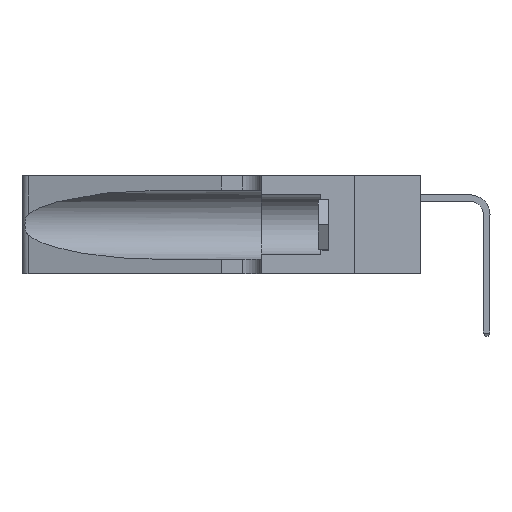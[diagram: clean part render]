
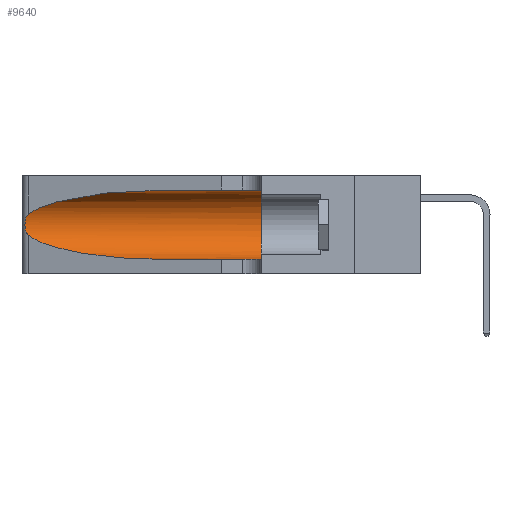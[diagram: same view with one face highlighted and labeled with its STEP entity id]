
A CAD part, left-side view. The second image highlights one B-rep face of the part: STEP entity #9640.
In plain terms, the highlighted cylindrical face has radius 3.308 mm (diameter 6.617 mm), a partial arc.
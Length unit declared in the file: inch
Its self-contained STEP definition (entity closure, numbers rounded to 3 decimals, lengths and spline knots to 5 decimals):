
#336 = CARTESIAN_POINT ( 'NONE',  ( 0.25487, 1.22718, 0.22369 ) ) ;
#427 = DIRECTION ( 'NONE',  ( 0., 0., 1. ) ) ;
#864 = CARTESIAN_POINT ( 'NONE',  ( 0.25487, 1.22718, 0.22369 ) ) ;
#1124 = AXIS2_PLACEMENT_3D ( 'NONE', #34029, #17379, #427 ) ;
#2568 = CARTESIAN_POINT ( 'NONE',  ( 0.25789, 1.23486, 0.15765 ) ) ;
#3024 = EDGE_CURVE ( 'NONE', #29465, #32838, #11775, .T. ) ;
#3069 = CARTESIAN_POINT ( 'NONE',  ( 0.1305, 0.72297, 0.31525 ) ) ;
#4039 = CARTESIAN_POINT ( 'NONE',  ( 0.1305, 0.72297, 0.05475 ) ) ;
#4772 = CARTESIAN_POINT ( 'NONE',  ( 0.1305, 0.72297, 0.05475 ) ) ;
#4785 = VECTOR ( 'NONE', #34734, 39.37008 ) ;
#5292 = CARTESIAN_POINT ( 'NONE',  ( 0.25555, 1.22994, 0.2215 ) ) ;
#5407 = CARTESIAN_POINT ( 'NONE',  ( 0.25555, 1.22993, 0.14849 ) ) ;
#6448 = ORIENTED_EDGE ( 'NONE', *, *, #29669, .T. ) ;
#6559 = CIRCLE ( 'NONE', #1124, 0.13025 ) ;
#8004 = CARTESIAN_POINT ( 'NONE',  ( 0.25487, 1.22718, 0.22369 ) ) ;
#8681 = ORIENTED_EDGE ( 'NONE', *, *, #9559, .F. ) ;
#8754 = CARTESIAN_POINT ( 'NONE',  ( 0.18966, 0.96281, 0.31525 ) ) ;
#9010 = VERTEX_POINT ( 'NONE', #864 ) ;
#9559 = EDGE_CURVE ( 'NONE', #32838, #14197, #6559, .T. ) ;
#9619 = CARTESIAN_POINT ( 'NONE',  ( 0.2373, 1.15595, 0.08982 ) ) ;
#9640 = ADVANCED_FACE ( 'NONE', ( #32488 ), #10149, .F. ) ;
#10149 = CYLINDRICAL_SURFACE ( 'NONE', #16273, 0.13025 ) ;
#10292 = EDGE_CURVE ( 'NONE', #32568, #14197, #32848, .T. ) ;
#10497 = DIRECTION ( 'NONE',  ( 0., -1., 0. ) ) ;
#10960 = CARTESIAN_POINT ( 'NONE',  ( 0.25787, 1.23484, 0.2124 ) ) ;
#11775 = LINE ( 'NONE', #19025, #25821 ) ;
#12058 = CARTESIAN_POINT ( 'NONE',  ( 0.1305, 1.61858, 0.185 ) ) ;
#13831 = CARTESIAN_POINT ( 'NONE',  ( 0.26018, 1.23835, 0.19895 ) ) ;
#14197 = VERTEX_POINT ( 'NONE', #29158 ) ;
#16273 = AXIS2_PLACEMENT_3D ( 'NONE', #12058, #31618, #26050 ) ;
#16666 = CARTESIAN_POINT ( 'NONE',  ( 0.26075, 1.23896, 0.178 ) ) ;
#16757 =( BOUNDED_CURVE ( )  B_SPLINE_CURVE ( 3, ( #3069, #8754, #17287, #336 ),
 .UNSPECIFIED., .F., .T. ) 
 B_SPLINE_CURVE_WITH_KNOTS ( ( 4, 4 ),
 ( 1.5708, 2.84003 ),
 .UNSPECIFIED. ) 
 CURVE ( )  GEOMETRIC_REPRESENTATION_ITEM ( )  RATIONAL_B_SPLINE_CURVE ( ( 1., 0.87, 0.87, 1. ) ) 
 REPRESENTATION_ITEM ( '' )  );
#17287 = CARTESIAN_POINT ( 'NONE',  ( 0.2373, 1.15595, 0.28018 ) ) ;
#17379 = DIRECTION ( 'NONE',  ( 0., 1., 0. ) ) ;
#17400 = ORIENTED_EDGE ( 'NONE', *, *, #22391, .T. ) ;
#19025 = CARTESIAN_POINT ( 'NONE',  ( 0.1305, 1.61858, 0.31525 ) ) ;
#19323 = EDGE_CURVE ( 'NONE', #9010, #26788, #35095, .T. ) ;
#19490 = CARTESIAN_POINT ( 'NONE',  ( 0.25856, 1.23593, 0.16098 ) ) ;
#20527 =( BOUNDED_CURVE ( )  B_SPLINE_CURVE ( 3, ( #32010, #9619, #20956, #4039 ),
 .UNSPECIFIED., .F., .F. ) 
 B_SPLINE_CURVE_WITH_KNOTS ( ( 4, 4 ),
 ( 3.44316, 4.71239 ),
 .UNSPECIFIED. ) 
 CURVE ( )  GEOMETRIC_REPRESENTATION_ITEM ( )  RATIONAL_B_SPLINE_CURVE ( ( 1., 0.87, 0.87, 1. ) ) 
 REPRESENTATION_ITEM ( '' )  );
#20602 = ORIENTED_EDGE ( 'NONE', *, *, #3024, .F. ) ;
#20956 = CARTESIAN_POINT ( 'NONE',  ( 0.18966, 0.96281, 0.05475 ) ) ;
#22290 = CARTESIAN_POINT ( 'NONE',  ( 0.25639, 1.23186, 0.15144 ) ) ;
#22391 = EDGE_CURVE ( 'NONE', #29465, #9010, #16757, .T. ) ;
#22992 = EDGE_LOOP ( 'NONE', ( #17400, #27299, #6448, #25802, #8681, #20602 ) ) ;
#24677 = CARTESIAN_POINT ( 'NONE',  ( 0.25487, 1.22718, 0.14631 ) ) ;
#25096 = CARTESIAN_POINT ( 'NONE',  ( 0.25487, 1.22718, 0.14631 ) ) ;
#25802 = ORIENTED_EDGE ( 'NONE', *, *, #10292, .T. ) ;
#25821 = VECTOR ( 'NONE', #10497, 39.37008 ) ;
#26050 = DIRECTION ( 'NONE',  ( 0., 0., -1. ) ) ;
#26788 = VERTEX_POINT ( 'NONE', #24677 ) ;
#27299 = ORIENTED_EDGE ( 'NONE', *, *, #19323, .T. ) ;
#27785 = CARTESIAN_POINT ( 'NONE',  ( 0.25639, 1.23184, 0.21858 ) ) ;
#29158 = CARTESIAN_POINT ( 'NONE',  ( 0.1305, 0.35, 0.05475 ) ) ;
#29465 = VERTEX_POINT ( 'NONE', #33925 ) ;
#29669 = EDGE_CURVE ( 'NONE', #26788, #32568, #20527, .T. ) ;
#30566 = CARTESIAN_POINT ( 'NONE',  ( 0.25854, 1.2359, 0.20912 ) ) ;
#31618 = DIRECTION ( 'NONE',  ( 0., -1., 0. ) ) ;
#31962 = CARTESIAN_POINT ( 'NONE',  ( 0.1305, 1.61858, 0.05475 ) ) ;
#32010 = CARTESIAN_POINT ( 'NONE',  ( 0.25487, 1.22718, 0.14631 ) ) ;
#32488 = FACE_OUTER_BOUND ( 'NONE', #22992, .T. ) ;
#32568 = VERTEX_POINT ( 'NONE', #4772 ) ;
#32838 = VERTEX_POINT ( 'NONE', #34018 ) ;
#32848 = LINE ( 'NONE', #31962, #4785 ) ;
#33334 = CARTESIAN_POINT ( 'NONE',  ( 0.26075, 1.23896, 0.19203 ) ) ;
#33925 = CARTESIAN_POINT ( 'NONE',  ( 0.1305, 0.72297, 0.31525 ) ) ;
#34018 = CARTESIAN_POINT ( 'NONE',  ( 0.1305, 0.35, 0.31525 ) ) ;
#34029 = CARTESIAN_POINT ( 'NONE',  ( 0.1305, 0.35, 0.185 ) ) ;
#34734 = DIRECTION ( 'NONE',  ( 0., -1., 0. ) ) ;
#35095 = B_SPLINE_CURVE_WITH_KNOTS ( 'NONE', 3,
 ( #8004, #5292, #27785, #10960, #30566, #13831, #33334, #16666, #36119, #19490, #2568, #22290, #5407, #25096 ),
 .UNSPECIFIED., .F., .F.,
 ( 4, 2, 2, 2, 2, 2, 4 ),
 ( 0., 0.00027, 0.00053, 0.00107, 0.0016, 0.00187, 0.00214 ),
 .UNSPECIFIED. ) ;
#36119 = CARTESIAN_POINT ( 'NONE',  ( 0.26017, 1.23833, 0.17102 ) ) ;
